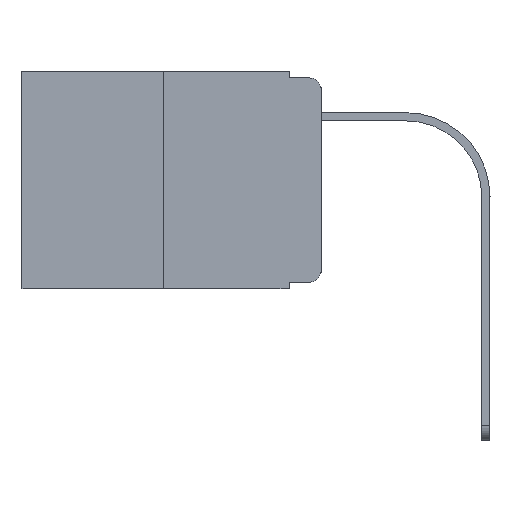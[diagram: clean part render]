
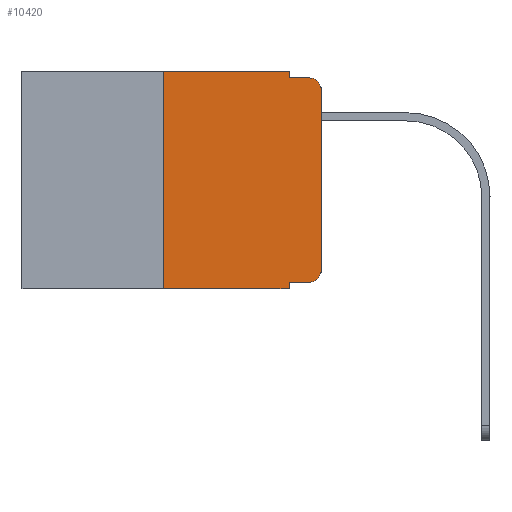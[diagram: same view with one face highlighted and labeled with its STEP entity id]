
A CAD part, left-side view. The second image highlights one B-rep face of the part: STEP entity #10420.
In plain terms, the highlighted planar face has unit normal (-1, 0, 0).
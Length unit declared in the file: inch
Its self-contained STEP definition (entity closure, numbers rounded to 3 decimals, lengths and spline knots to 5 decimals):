
#251 = CARTESIAN_POINT ( 'NONE',  ( 0., 0.25, 0. ) ) ;
#332 = DIRECTION ( 'NONE',  ( 0., 0., -1. ) ) ;
#557 = EDGE_CURVE ( 'NONE', #9214, #16972, #11224, .T. ) ;
#562 = ORIENTED_EDGE ( 'NONE', *, *, #9245, .T. ) ;
#1215 = DIRECTION ( 'NONE',  ( 0., 0., -1. ) ) ;
#1595 = DIRECTION ( 'NONE',  ( 0., 0., -1. ) ) ;
#1655 = ORIENTED_EDGE ( 'NONE', *, *, #5629, .F. ) ;
#1815 = LINE ( 'NONE', #251, #6982 ) ;
#2112 = EDGE_LOOP ( 'NONE', ( #562, #6595, #1655, #17257, #4587, #15354, #19450, #6325, #10322, #4184 ) ) ;
#2309 = CARTESIAN_POINT ( 'NONE',  ( 0., 0.02, -0.01 ) ) ;
#2390 = AXIS2_PLACEMENT_3D ( 'NONE', #14700, #19620, #17937 ) ;
#2907 = CIRCLE ( 'NONE', #5246, 0.02 ) ;
#4184 = ORIENTED_EDGE ( 'NONE', *, *, #557, .T. ) ;
#4201 = LINE ( 'NONE', #10386, #11121 ) ;
#4332 = LINE ( 'NONE', #4531, #13977 ) ;
#4393 = VERTEX_POINT ( 'NONE', #13029 ) ;
#4531 = CARTESIAN_POINT ( 'NONE',  ( 0., 0.473, -0.343 ) ) ;
#4587 = ORIENTED_EDGE ( 'NONE', *, *, #8843, .F. ) ;
#4963 = VERTEX_POINT ( 'NONE', #8637 ) ;
#5239 = LINE ( 'NONE', #18014, #12004 ) ;
#5246 = AXIS2_PLACEMENT_3D ( 'NONE', #11055, #15858, #1215 ) ;
#5617 = CARTESIAN_POINT ( 'NONE',  ( 0., 0., -0.313 ) ) ;
#5629 = EDGE_CURVE ( 'NONE', #13602, #7544, #12383, .T. ) ;
#5677 = LINE ( 'NONE', #12077, #8764 ) ;
#5703 = VECTOR ( 'NONE', #8489, 39.37008 ) ;
#5960 = VECTOR ( 'NONE', #11838, 39.37008 ) ;
#6058 = VECTOR ( 'NONE', #7536, 39.37008 ) ;
#6325 = ORIENTED_EDGE ( 'NONE', *, *, #7601, .F. ) ;
#6595 = ORIENTED_EDGE ( 'NONE', *, *, #16216, .T. ) ;
#6911 = LINE ( 'NONE', #8389, #5703 ) ;
#6982 = VECTOR ( 'NONE', #8700, 39.37008 ) ;
#7033 = EDGE_CURVE ( 'NONE', #7511, #15149, #1815, .T. ) ;
#7126 = DIRECTION ( 'NONE',  ( 0., -1., 0. ) ) ;
#7239 = CARTESIAN_POINT ( 'NONE',  ( 0., 0.051, -0.01 ) ) ;
#7511 = VERTEX_POINT ( 'NONE', #19591 ) ;
#7536 = DIRECTION ( 'NONE',  ( 0., -1., 0. ) ) ;
#7543 = CARTESIAN_POINT ( 'NONE',  ( 0., 0.051, -0.333 ) ) ;
#7544 = VERTEX_POINT ( 'NONE', #2309 ) ;
#7575 = EDGE_CURVE ( 'NONE', #12089, #9214, #11428, .T. ) ;
#7601 = EDGE_CURVE ( 'NONE', #12089, #4963, #5239, .T. ) ;
#8389 = CARTESIAN_POINT ( 'NONE',  ( 0., 0.051, 0. ) ) ;
#8489 = DIRECTION ( 'NONE',  ( 0., 0., -1. ) ) ;
#8637 = CARTESIAN_POINT ( 'NONE',  ( 0., 0.051, -0.343 ) ) ;
#8700 = DIRECTION ( 'NONE',  ( 0., 0., 1. ) ) ;
#8764 = VECTOR ( 'NONE', #7126, 39.37008 ) ;
#8843 = EDGE_CURVE ( 'NONE', #15149, #13500, #5677, .T. ) ;
#9214 = VERTEX_POINT ( 'NONE', #17718 ) ;
#9245 = EDGE_CURVE ( 'NONE', #16972, #4393, #4201, .T. ) ;
#9537 = CARTESIAN_POINT ( 'NONE',  ( 0., 0.02, -0.313 ) ) ;
#10322 = ORIENTED_EDGE ( 'NONE', *, *, #7575, .T. ) ;
#10386 = CARTESIAN_POINT ( 'NONE',  ( 0., 0., 0. ) ) ;
#10420 = ADVANCED_FACE ( 'NONE', ( #13011 ), #14804, .F. ) ;
#10467 = EDGE_CURVE ( 'NONE', #13500, #13602, #6911, .T. ) ;
#11055 = CARTESIAN_POINT ( 'NONE',  ( 0., 0.02, -0.03 ) ) ;
#11121 = VECTOR ( 'NONE', #19910, 39.37008 ) ;
#11224 = CIRCLE ( 'NONE', #11910, 0.02 ) ;
#11428 = LINE ( 'NONE', #13099, #5960 ) ;
#11838 = DIRECTION ( 'NONE',  ( 0., -1., 0. ) ) ;
#11910 = AXIS2_PLACEMENT_3D ( 'NONE', #9537, #19287, #1595 ) ;
#12004 = VECTOR ( 'NONE', #332, 39.37008 ) ;
#12077 = CARTESIAN_POINT ( 'NONE',  ( 0., 0.473, 0. ) ) ;
#12089 = VERTEX_POINT ( 'NONE', #7543 ) ;
#12383 = LINE ( 'NONE', #7239, #6058 ) ;
#13011 = FACE_OUTER_BOUND ( 'NONE', #2112, .T. ) ;
#13029 = CARTESIAN_POINT ( 'NONE',  ( 0., 0., -0.03 ) ) ;
#13099 = CARTESIAN_POINT ( 'NONE',  ( 0., 0.051, -0.333 ) ) ;
#13500 = VERTEX_POINT ( 'NONE', #16595 ) ;
#13602 = VERTEX_POINT ( 'NONE', #18561 ) ;
#13977 = VECTOR ( 'NONE', #14076, 39.37008 ) ;
#14076 = DIRECTION ( 'NONE',  ( 0., -1., 0. ) ) ;
#14700 = CARTESIAN_POINT ( 'NONE',  ( 0., 0.473, 0. ) ) ;
#14804 = PLANE ( 'NONE',  #2390 ) ;
#15149 = VERTEX_POINT ( 'NONE', #15399 ) ;
#15354 = ORIENTED_EDGE ( 'NONE', *, *, #7033, .F. ) ;
#15399 = CARTESIAN_POINT ( 'NONE',  ( 0., 0.25, 0. ) ) ;
#15858 = DIRECTION ( 'NONE',  ( -1., 0., 0. ) ) ;
#16216 = EDGE_CURVE ( 'NONE', #4393, #7544, #2907, .T. ) ;
#16595 = CARTESIAN_POINT ( 'NONE',  ( 0., 0.051, 0. ) ) ;
#16602 = EDGE_CURVE ( 'NONE', #7511, #4963, #4332, .T. ) ;
#16972 = VERTEX_POINT ( 'NONE', #5617 ) ;
#17257 = ORIENTED_EDGE ( 'NONE', *, *, #10467, .F. ) ;
#17718 = CARTESIAN_POINT ( 'NONE',  ( 0., 0.02, -0.333 ) ) ;
#17937 = DIRECTION ( 'NONE',  ( 0., 0., -1. ) ) ;
#18014 = CARTESIAN_POINT ( 'NONE',  ( 0., 0.051, 0. ) ) ;
#18561 = CARTESIAN_POINT ( 'NONE',  ( 0., 0.051, -0.01 ) ) ;
#19287 = DIRECTION ( 'NONE',  ( -1., 0., 0. ) ) ;
#19450 = ORIENTED_EDGE ( 'NONE', *, *, #16602, .T. ) ;
#19591 = CARTESIAN_POINT ( 'NONE',  ( 0., 0.25, -0.343 ) ) ;
#19620 = DIRECTION ( 'NONE',  ( 1., 0., 0. ) ) ;
#19910 = DIRECTION ( 'NONE',  ( 0., 0., 1. ) ) ;
